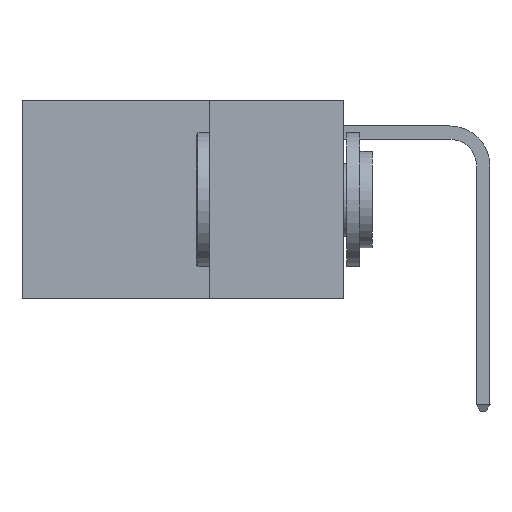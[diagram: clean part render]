
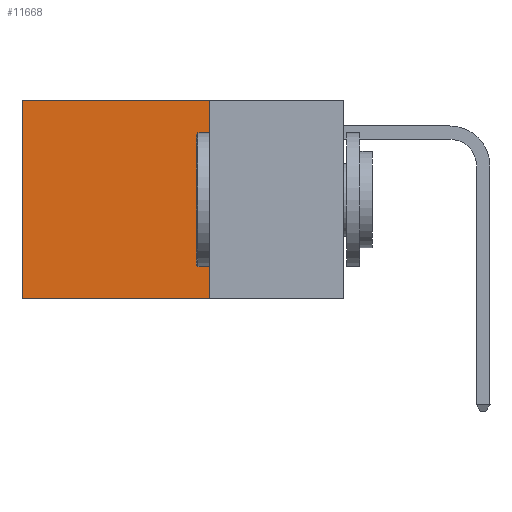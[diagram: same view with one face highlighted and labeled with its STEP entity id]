
A CAD part, left-side view. The second image highlights one B-rep face of the part: STEP entity #11668.
In plain terms, the highlighted planar face has unit normal (-1, 0, 0).
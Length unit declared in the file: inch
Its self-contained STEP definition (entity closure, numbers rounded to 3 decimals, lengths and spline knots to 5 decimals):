
#895 = CARTESIAN_POINT ( 'NONE',  ( 0.2625, 0.6, -0.37 ) ) ;
#1090 = ORIENTED_EDGE ( 'NONE', *, *, #9856, .T. ) ;
#1507 = VERTEX_POINT ( 'NONE', #9601 ) ;
#1928 = EDGE_CURVE ( 'NONE', #11377, #6426, #5093, .T. ) ;
#2206 = ORIENTED_EDGE ( 'NONE', *, *, #1928, .F. ) ;
#2265 = VECTOR ( 'NONE', #7541, 39.37008 ) ;
#2281 = AXIS2_PLACEMENT_3D ( 'NONE', #7324, #2922, #10918 ) ;
#2514 = CARTESIAN_POINT ( 'NONE',  ( 0.2625, 0.25, 0. ) ) ;
#2922 = DIRECTION ( 'NONE',  ( 1., 0., 0. ) ) ;
#3136 = CARTESIAN_POINT ( 'NONE',  ( 0.2625, 0.6, 0. ) ) ;
#3352 = DIRECTION ( 'NONE',  ( 0., 1., 0. ) ) ;
#3531 = LINE ( 'NONE', #2514, #10966 ) ;
#3820 = PLANE ( 'NONE',  #2281 ) ;
#4126 = CARTESIAN_POINT ( 'NONE',  ( 0.2625, 0.25, 0. ) ) ;
#4715 = ORIENTED_EDGE ( 'NONE', *, *, #9230, .T. ) ;
#4751 = LINE ( 'NONE', #4126, #9652 ) ;
#5093 = LINE ( 'NONE', #10361, #8534 ) ;
#6426 = VERTEX_POINT ( 'NONE', #895 ) ;
#6710 = LINE ( 'NONE', #3136, #2265 ) ;
#6731 = ORIENTED_EDGE ( 'NONE', *, *, #9803, .F. ) ;
#7324 = CARTESIAN_POINT ( 'NONE',  ( 0.2625, 0.25, 0. ) ) ;
#7398 = CARTESIAN_POINT ( 'NONE',  ( 0.2625, 0.25, -0.37 ) ) ;
#7488 = CARTESIAN_POINT ( 'NONE',  ( 0.2625, 0.6, 0. ) ) ;
#7541 = DIRECTION ( 'NONE',  ( 0., 0., -1. ) ) ;
#7888 = DIRECTION ( 'NONE',  ( 0., 1., 0. ) ) ;
#8266 = FACE_OUTER_BOUND ( 'NONE', #11603, .T. ) ;
#8534 = VECTOR ( 'NONE', #7888, 39.37008 ) ;
#9230 = EDGE_CURVE ( 'NONE', #10393, #6426, #6710, .T. ) ;
#9601 = CARTESIAN_POINT ( 'NONE',  ( 0.2625, 0.25, 0. ) ) ;
#9652 = VECTOR ( 'NONE', #10465, 39.37008 ) ;
#9803 = EDGE_CURVE ( 'NONE', #1507, #11377, #4751, .T. ) ;
#9856 = EDGE_CURVE ( 'NONE', #1507, #10393, #3531, .T. ) ;
#10361 = CARTESIAN_POINT ( 'NONE',  ( 0.2625, 0.25, -0.37 ) ) ;
#10393 = VERTEX_POINT ( 'NONE', #7488 ) ;
#10465 = DIRECTION ( 'NONE',  ( 0., 0., -1. ) ) ;
#10918 = DIRECTION ( 'NONE',  ( 0., 0., -1. ) ) ;
#10966 = VECTOR ( 'NONE', #3352, 39.37008 ) ;
#11377 = VERTEX_POINT ( 'NONE', #7398 ) ;
#11603 = EDGE_LOOP ( 'NONE', ( #4715, #2206, #6731, #1090 ) ) ;
#11668 = ADVANCED_FACE ( 'NONE', ( #8266 ), #3820, .F. ) ;
